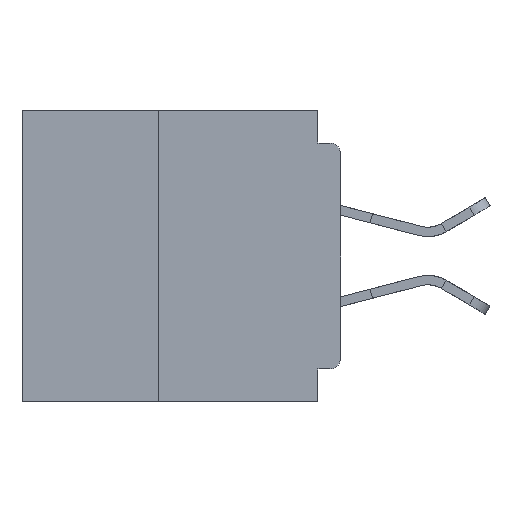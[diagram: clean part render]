
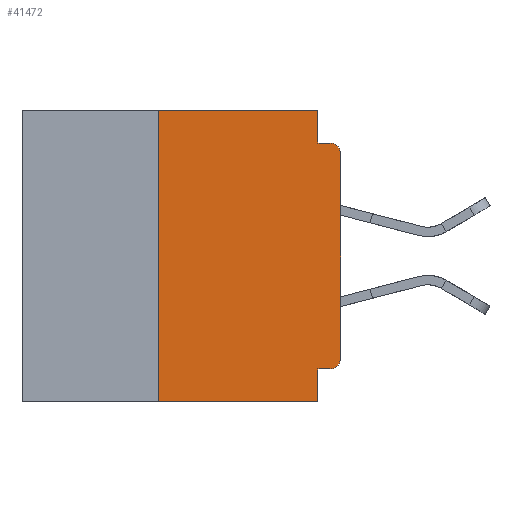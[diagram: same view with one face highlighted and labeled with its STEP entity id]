
A CAD part, left-side view. The second image highlights one B-rep face of the part: STEP entity #41472.
In plain terms, the highlighted planar face has unit normal (-1, 0, 0).
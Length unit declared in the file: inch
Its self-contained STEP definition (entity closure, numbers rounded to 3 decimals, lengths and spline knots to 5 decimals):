
#21 = ORIENTED_EDGE ( 'NONE', *, *, #21514, .F. ) ;
#2044 = ORIENTED_EDGE ( 'NONE', *, *, #15920, .F. ) ;
#2180 = CARTESIAN_POINT ( 'NONE',  ( 0., 0.031, 0. ) ) ;
#3112 = EDGE_CURVE ( 'NONE', #3408, #34067, #5514, .T. ) ;
#3408 = VERTEX_POINT ( 'NONE', #4520 ) ;
#3570 = VERTEX_POINT ( 'NONE', #35842 ) ;
#3629 = EDGE_CURVE ( 'NONE', #34067, #32639, #29491, .T. ) ;
#4047 = ORIENTED_EDGE ( 'NONE', *, *, #29436, .T. ) ;
#4130 = LINE ( 'NONE', #32381, #30306 ) ;
#4520 = CARTESIAN_POINT ( 'NONE',  ( 0., 0.015, -0.355 ) ) ;
#5122 = CARTESIAN_POINT ( 'NONE',  ( 0., 0.25, -0.4 ) ) ;
#5163 = VERTEX_POINT ( 'NONE', #30550 ) ;
#5514 = LINE ( 'NONE', #26812, #22649 ) ;
#6198 = AXIS2_PLACEMENT_3D ( 'NONE', #19528, #42965, #22958 ) ;
#6388 = CARTESIAN_POINT ( 'NONE',  ( 0., 0., -0.34 ) ) ;
#6882 = ORIENTED_EDGE ( 'NONE', *, *, #23542, .F. ) ;
#7405 = CARTESIAN_POINT ( 'NONE',  ( 0., 0.015, -0.045 ) ) ;
#7969 = CARTESIAN_POINT ( 'NONE',  ( 0., 0.437, 0. ) ) ;
#8461 = CARTESIAN_POINT ( 'NONE',  ( 0., 0.437, 0. ) ) ;
#9824 = DIRECTION ( 'NONE',  ( 0., 1., 0. ) ) ;
#9901 = EDGE_CURVE ( 'NONE', #31027, #32639, #17305, .T. ) ;
#11439 = DIRECTION ( 'NONE',  ( 0., -1., 0. ) ) ;
#11927 = DIRECTION ( 'NONE',  ( 1., 0., 0. ) ) ;
#12013 = CARTESIAN_POINT ( 'NONE',  ( 0., 0.25, -0.4 ) ) ;
#12654 = CARTESIAN_POINT ( 'NONE',  ( 0., 0.031, -0.4 ) ) ;
#13266 = EDGE_CURVE ( 'NONE', #3408, #25696, #36066, .T. ) ;
#15920 = EDGE_CURVE ( 'NONE', #3570, #15951, #31610, .T. ) ;
#15951 = VERTEX_POINT ( 'NONE', #41749 ) ;
#16034 = VERTEX_POINT ( 'NONE', #18867 ) ;
#16726 = CARTESIAN_POINT ( 'NONE',  ( 0., 0.015, -0.06 ) ) ;
#17305 = LINE ( 'NONE', #18976, #25300 ) ;
#17423 = VERTEX_POINT ( 'NONE', #7405 ) ;
#17884 = VECTOR ( 'NONE', #29515, 39.37008 ) ;
#18867 = CARTESIAN_POINT ( 'NONE',  ( 0., 0., -0.06 ) ) ;
#18976 = CARTESIAN_POINT ( 'NONE',  ( 0., 0.437, -0.4 ) ) ;
#19230 = VECTOR ( 'NONE', #20533, 39.37008 ) ;
#19239 = CARTESIAN_POINT ( 'NONE',  ( 0., 0.031, -0.355 ) ) ;
#19400 = VECTOR ( 'NONE', #36271, 39.37008 ) ;
#19528 = CARTESIAN_POINT ( 'NONE',  ( 0., 0.015, -0.34 ) ) ;
#20163 = DIRECTION ( 'NONE',  ( 0., 0., -1. ) ) ;
#20293 = LINE ( 'NONE', #30598, #19230 ) ;
#20533 = DIRECTION ( 'NONE',  ( 0., 0., 1. ) ) ;
#20943 = ORIENTED_EDGE ( 'NONE', *, *, #35734, .T. ) ;
#20987 = ORIENTED_EDGE ( 'NONE', *, *, #3112, .F. ) ;
#21514 = EDGE_CURVE ( 'NONE', #15951, #5163, #34788, .T. ) ;
#22418 = DIRECTION ( 'NONE',  ( 0., -1., 0. ) ) ;
#22649 = VECTOR ( 'NONE', #9824, 39.37008 ) ;
#22958 = DIRECTION ( 'NONE',  ( 0., 0., -1. ) ) ;
#23542 = EDGE_CURVE ( 'NONE', #5163, #17423, #4130, .T. ) ;
#23840 = FACE_OUTER_BOUND ( 'NONE', #39126, .T. ) ;
#25300 = VECTOR ( 'NONE', #22418, 39.37008 ) ;
#25696 = VERTEX_POINT ( 'NONE', #6388 ) ;
#26812 = CARTESIAN_POINT ( 'NONE',  ( 0., 0., -0.355 ) ) ;
#28883 = PLANE ( 'NONE',  #29328 ) ;
#29328 = AXIS2_PLACEMENT_3D ( 'NONE', #8461, #11927, #35573 ) ;
#29436 = EDGE_CURVE ( 'NONE', #25696, #16034, #20293, .T. ) ;
#29491 = LINE ( 'NONE', #12654, #19400 ) ;
#29515 = DIRECTION ( 'NONE',  ( 0., 0., -1. ) ) ;
#29810 = EDGE_CURVE ( 'NONE', #31027, #3570, #40188, .T. ) ;
#30306 = VECTOR ( 'NONE', #35705, 39.37008 ) ;
#30550 = CARTESIAN_POINT ( 'NONE',  ( 0., 0.031, -0.045 ) ) ;
#30552 = VECTOR ( 'NONE', #11439, 39.37008 ) ;
#30598 = CARTESIAN_POINT ( 'NONE',  ( 0., 0., 0. ) ) ;
#31027 = VERTEX_POINT ( 'NONE', #5122 ) ;
#31389 = VECTOR ( 'NONE', #35655, 39.37008 ) ;
#31610 = LINE ( 'NONE', #7969, #30552 ) ;
#32381 = CARTESIAN_POINT ( 'NONE',  ( 0., 0., -0.045 ) ) ;
#32639 = VERTEX_POINT ( 'NONE', #34828 ) ;
#34067 = VERTEX_POINT ( 'NONE', #19239 ) ;
#34686 = ORIENTED_EDGE ( 'NONE', *, *, #13266, .T. ) ;
#34788 = LINE ( 'NONE', #2180, #17884 ) ;
#34828 = CARTESIAN_POINT ( 'NONE',  ( 0., 0.031, -0.4 ) ) ;
#35573 = DIRECTION ( 'NONE',  ( 0., 0., -1. ) ) ;
#35655 = DIRECTION ( 'NONE',  ( 0., 0., 1. ) ) ;
#35705 = DIRECTION ( 'NONE',  ( 0., -1., 0. ) ) ;
#35734 = EDGE_CURVE ( 'NONE', #16034, #17423, #36410, .T. ) ;
#35833 = ORIENTED_EDGE ( 'NONE', *, *, #29810, .F. ) ;
#35842 = CARTESIAN_POINT ( 'NONE',  ( 0., 0.25, 0. ) ) ;
#36066 = CIRCLE ( 'NONE', #6198, 0.015 ) ;
#36271 = DIRECTION ( 'NONE',  ( 0., 0., -1. ) ) ;
#36387 = ORIENTED_EDGE ( 'NONE', *, *, #9901, .T. ) ;
#36410 = CIRCLE ( 'NONE', #39170, 0.015 ) ;
#39126 = EDGE_LOOP ( 'NONE', ( #4047, #20943, #6882, #21, #2044, #35833, #36387, #39632, #20987, #34686 ) ) ;
#39170 = AXIS2_PLACEMENT_3D ( 'NONE', #16726, #40236, #20163 ) ;
#39632 = ORIENTED_EDGE ( 'NONE', *, *, #3629, .F. ) ;
#40188 = LINE ( 'NONE', #12013, #31389 ) ;
#40236 = DIRECTION ( 'NONE',  ( -1., 0., 0. ) ) ;
#41472 = ADVANCED_FACE ( 'NONE', ( #23840 ), #28883, .F. ) ;
#41749 = CARTESIAN_POINT ( 'NONE',  ( 0., 0.031, 0. ) ) ;
#42965 = DIRECTION ( 'NONE',  ( -1., 0., 0. ) ) ;
